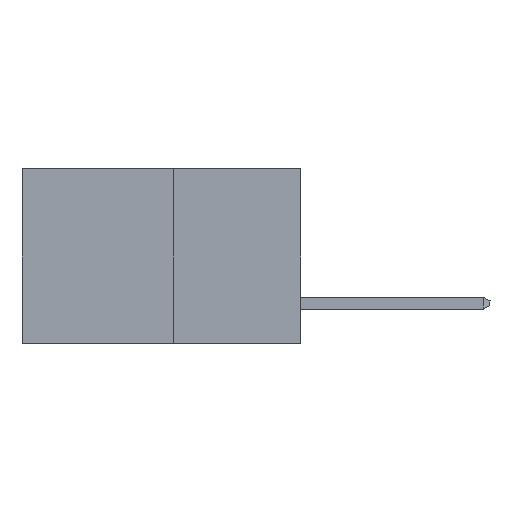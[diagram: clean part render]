
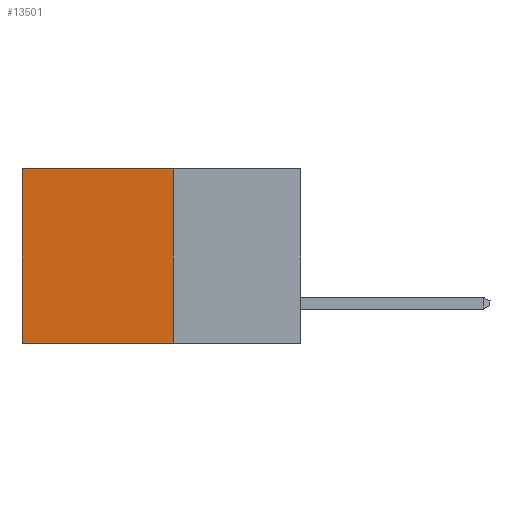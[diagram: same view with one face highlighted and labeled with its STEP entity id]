
A CAD part, left-side view. The second image highlights one B-rep face of the part: STEP entity #13501.
In plain terms, the highlighted planar face has unit normal (-1, 0, 0).
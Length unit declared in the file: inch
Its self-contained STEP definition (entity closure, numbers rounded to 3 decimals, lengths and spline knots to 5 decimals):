
#378 = DIRECTION ( 'NONE',  ( 1., 0., 0. ) ) ;
#649 = CARTESIAN_POINT ( 'NONE',  ( 0.277, 0.27, -0.37 ) ) ;
#770 = VERTEX_POINT ( 'NONE', #2040 ) ;
#1729 = ORIENTED_EDGE ( 'NONE', *, *, #15177, .T. ) ;
#2040 = CARTESIAN_POINT ( 'NONE',  ( 0.277, 0.27, 0. ) ) ;
#2726 = EDGE_CURVE ( 'NONE', #4288, #3735, #6453, .T. ) ;
#2729 = EDGE_CURVE ( 'NONE', #770, #4288, #3642, .T. ) ;
#3265 = VECTOR ( 'NONE', #4431, 39.37008 ) ;
#3642 = LINE ( 'NONE', #4113, #12875 ) ;
#3735 = VERTEX_POINT ( 'NONE', #8575 ) ;
#4005 = VECTOR ( 'NONE', #11633, 39.37008 ) ;
#4113 = CARTESIAN_POINT ( 'NONE',  ( 0.277, 0.27, -0.37 ) ) ;
#4133 = DIRECTION ( 'NONE',  ( 0., 0., -1. ) ) ;
#4288 = VERTEX_POINT ( 'NONE', #649 ) ;
#4342 = CARTESIAN_POINT ( 'NONE',  ( 0.277, 0.27, -0.37 ) ) ;
#4427 = CARTESIAN_POINT ( 'NONE',  ( 0.277, 0.59, -0.37 ) ) ;
#4431 = DIRECTION ( 'NONE',  ( 0., 1., 0. ) ) ;
#5217 = CARTESIAN_POINT ( 'NONE',  ( 0.277, 0.59, 0. ) ) ;
#5257 = AXIS2_PLACEMENT_3D ( 'NONE', #12427, #378, #8833 ) ;
#5432 = DIRECTION ( 'NONE',  ( 0., 1., 0. ) ) ;
#6164 = VERTEX_POINT ( 'NONE', #5217 ) ;
#6453 = LINE ( 'NONE', #4342, #3265 ) ;
#7645 = VECTOR ( 'NONE', #5432, 39.37008 ) ;
#7891 = EDGE_CURVE ( 'NONE', #770, #6164, #8005, .T. ) ;
#8005 = LINE ( 'NONE', #11492, #7645 ) ;
#8575 = CARTESIAN_POINT ( 'NONE',  ( 0.277, 0.59, -0.37 ) ) ;
#8769 = EDGE_LOOP ( 'NONE', ( #1729, #14533, #12528, #9700 ) ) ;
#8833 = DIRECTION ( 'NONE',  ( 0., 0., -1. ) ) ;
#9337 = FACE_OUTER_BOUND ( 'NONE', #8769, .T. ) ;
#9700 = ORIENTED_EDGE ( 'NONE', *, *, #7891, .T. ) ;
#11492 = CARTESIAN_POINT ( 'NONE',  ( 0.277, 0.27, 0. ) ) ;
#11633 = DIRECTION ( 'NONE',  ( 0., 0., -1. ) ) ;
#12427 = CARTESIAN_POINT ( 'NONE',  ( 0.277, 0.27, -0.37 ) ) ;
#12528 = ORIENTED_EDGE ( 'NONE', *, *, #2729, .F. ) ;
#12875 = VECTOR ( 'NONE', #4133, 39.37008 ) ;
#13501 = ADVANCED_FACE ( 'NONE', ( #9337 ), #14774, .F. ) ;
#13960 = LINE ( 'NONE', #4427, #4005 ) ;
#14533 = ORIENTED_EDGE ( 'NONE', *, *, #2726, .F. ) ;
#14774 = PLANE ( 'NONE',  #5257 ) ;
#15177 = EDGE_CURVE ( 'NONE', #6164, #3735, #13960, .T. ) ;
